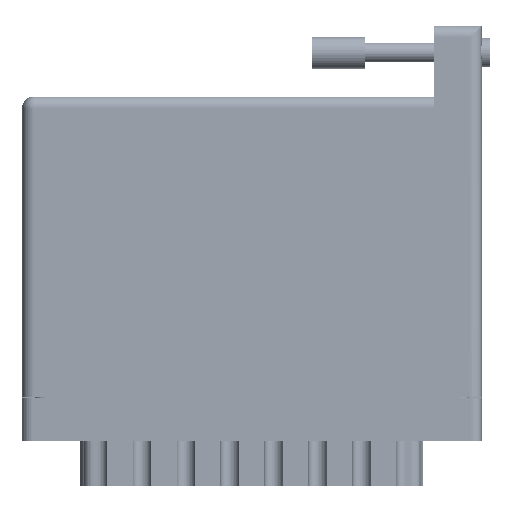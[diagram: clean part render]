
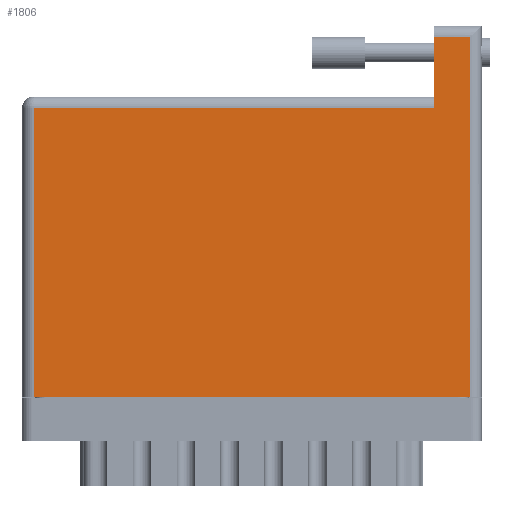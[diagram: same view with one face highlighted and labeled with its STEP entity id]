
A CAD part, front view. The second image highlights one B-rep face of the part: STEP entity #1806.
In plain terms, the highlighted face is planar.
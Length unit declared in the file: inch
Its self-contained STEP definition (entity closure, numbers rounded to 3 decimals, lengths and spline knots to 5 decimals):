
#1806 = ADVANCED_FACE ( 'NONE', ( #25743 ), #42510, .F. ) ;
#1831 = LINE ( 'NONE', #59156, #18509 ) ;
#3461 = ORIENTED_EDGE ( 'NONE', *, *, #18982, .T. ) ;
#4020 = DIRECTION ( 'NONE',  ( 0., -1., 0. ) ) ;
#4745 = DIRECTION ( 'NONE',  ( 1., 0., 0. ) ) ;
#5514 = EDGE_CURVE ( 'NONE', #50074, #20479, #28632, .T. ) ;
#10868 = VECTOR ( 'NONE', #4020, 39.37008 ) ;
#11949 = VERTEX_POINT ( 'NONE', #12768 ) ;
#12063 = EDGE_CURVE ( 'NONE', #20479, #60181, #1831, .T. ) ;
#12768 = CARTESIAN_POINT ( 'NONE',  ( 2.438, 1.705, 0. ) ) ;
#12796 = CARTESIAN_POINT ( 'NONE',  ( 2.438, 2.125, 0. ) ) ;
#12960 = CARTESIAN_POINT ( 'NONE',  ( 0., 2.125, 0. ) ) ;
#13857 = AXIS2_PLACEMENT_3D ( 'NONE', #47685, #31035, #59736 ) ;
#15191 = ORIENTED_EDGE ( 'NONE', *, *, #64682, .T. ) ;
#16388 = ORIENTED_EDGE ( 'NONE', *, *, #5514, .T. ) ;
#18509 = VECTOR ( 'NONE', #36535, 39.37008 ) ;
#18982 = EDGE_CURVE ( 'NONE', #11949, #30487, #42834, .T. ) ;
#20091 = CARTESIAN_POINT ( 'NONE',  ( 2.648, 2.125, 0. ) ) ;
#20479 = VERTEX_POINT ( 'NONE', #52460 ) ;
#21608 = VERTEX_POINT ( 'NONE', #12796 ) ;
#25743 = FACE_OUTER_BOUND ( 'NONE', #68289, .T. ) ;
#26158 = CARTESIAN_POINT ( 'NONE',  ( 0., 1.705, 0. ) ) ;
#28632 = LINE ( 'NONE', #54304, #60206 ) ;
#30487 = VERTEX_POINT ( 'NONE', #40819 ) ;
#31035 = DIRECTION ( 'NONE',  ( 0., 0., -1. ) ) ;
#31067 = VECTOR ( 'NONE', #48401, 39.37008 ) ;
#31992 = DIRECTION ( 'NONE',  ( -1., 0., 0. ) ) ;
#36535 = DIRECTION ( 'NONE',  ( 0., 1., 0. ) ) ;
#40229 = VECTOR ( 'NONE', #31992, 39.37008 ) ;
#40819 = CARTESIAN_POINT ( 'NONE',  ( 0.07, 1.705, 0. ) ) ;
#42510 = PLANE ( 'NONE',  #13857 ) ;
#42834 = LINE ( 'NONE', #26158, #40229 ) ;
#45347 = CARTESIAN_POINT ( 'NONE',  ( 0.07, 0., 0. ) ) ;
#46524 = DIRECTION ( 'NONE',  ( -1., 0., 0. ) ) ;
#47188 = LINE ( 'NONE', #12960, #48949 ) ;
#47685 = CARTESIAN_POINT ( 'NONE',  ( 0., 1.775, 0. ) ) ;
#48401 = DIRECTION ( 'NONE',  ( 0., -1., 0. ) ) ;
#48949 = VECTOR ( 'NONE', #46524, 39.37008 ) ;
#50074 = VERTEX_POINT ( 'NONE', #45347 ) ;
#51234 = LINE ( 'NONE', #54307, #31067 ) ;
#52460 = CARTESIAN_POINT ( 'NONE',  ( 2.648, 0., 0. ) ) ;
#54304 = CARTESIAN_POINT ( 'NONE',  ( 0., 0., 0. ) ) ;
#54307 = CARTESIAN_POINT ( 'NONE',  ( 0.07, 0., 0. ) ) ;
#57433 = LINE ( 'NONE', #71942, #10868 ) ;
#57855 = ORIENTED_EDGE ( 'NONE', *, *, #12063, .T. ) ;
#59156 = CARTESIAN_POINT ( 'NONE',  ( 2.648, 2.195, 0. ) ) ;
#59554 = ORIENTED_EDGE ( 'NONE', *, *, #61923, .T. ) ;
#59736 = DIRECTION ( 'NONE',  ( -1., 0., 0. ) ) ;
#59810 = ORIENTED_EDGE ( 'NONE', *, *, #72193, .T. ) ;
#60181 = VERTEX_POINT ( 'NONE', #20091 ) ;
#60206 = VECTOR ( 'NONE', #4745, 39.37008 ) ;
#61923 = EDGE_CURVE ( 'NONE', #60181, #21608, #47188, .T. ) ;
#64682 = EDGE_CURVE ( 'NONE', #30487, #50074, #51234, .T. ) ;
#68289 = EDGE_LOOP ( 'NONE', ( #3461, #15191, #16388, #57855, #59554, #59810 ) ) ;
#71942 = CARTESIAN_POINT ( 'NONE',  ( 2.438, 2.195, 0. ) ) ;
#72193 = EDGE_CURVE ( 'NONE', #21608, #11949, #57433, .T. ) ;
